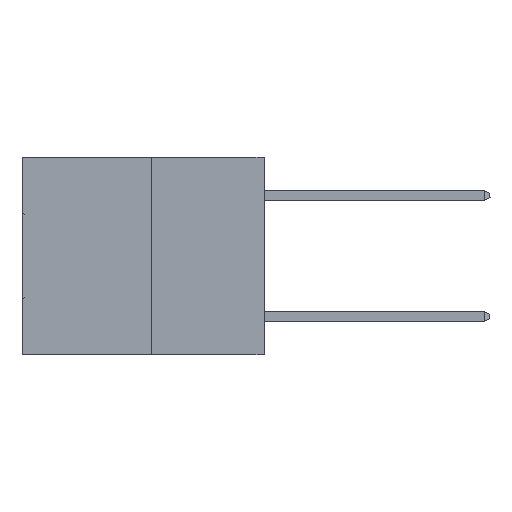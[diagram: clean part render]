
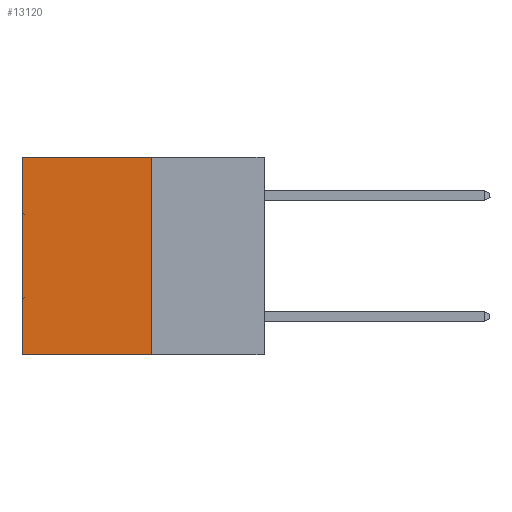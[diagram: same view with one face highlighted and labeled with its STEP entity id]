
A CAD part, left-side view. The second image highlights one B-rep face of the part: STEP entity #13120.
In plain terms, the highlighted planar face has unit normal (-1, 0, 0).
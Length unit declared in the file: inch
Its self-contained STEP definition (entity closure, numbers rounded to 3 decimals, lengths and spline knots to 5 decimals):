
#228 = CARTESIAN_POINT ( 'NONE',  ( 0.3165, 0.28, -0.49 ) ) ;
#1295 = FACE_OUTER_BOUND ( 'NONE', #20181, .T. ) ;
#1435 = VECTOR ( 'NONE', #20917, 39.37008 ) ;
#1850 = LINE ( 'NONE', #34299, #25041 ) ;
#3273 = VERTEX_POINT ( 'NONE', #21828 ) ;
#4884 = VERTEX_POINT ( 'NONE', #9350 ) ;
#6890 = LINE ( 'NONE', #12494, #13400 ) ;
#7121 = EDGE_CURVE ( 'NONE', #3273, #4884, #6890, .T. ) ;
#8091 = VECTOR ( 'NONE', #23873, 39.37008 ) ;
#8576 = VERTEX_POINT ( 'NONE', #11749 ) ;
#9350 = CARTESIAN_POINT ( 'NONE',  ( 0.3165, 0.6, -0.49 ) ) ;
#9595 = DIRECTION ( 'NONE',  ( 1., 0., 0. ) ) ;
#9751 = LINE ( 'NONE', #228, #1435 ) ;
#10992 = CARTESIAN_POINT ( 'NONE',  ( 0.3165, 0.28, -0.49 ) ) ;
#11749 = CARTESIAN_POINT ( 'NONE',  ( 0.3165, 0.28, 0. ) ) ;
#12494 = CARTESIAN_POINT ( 'NONE',  ( 0.3165, 0.6, -0.49 ) ) ;
#13120 = ADVANCED_FACE ( 'NONE', ( #1295 ), #26601, .F. ) ;
#13400 = VECTOR ( 'NONE', #15300, 39.37008 ) ;
#15300 = DIRECTION ( 'NONE',  ( 0., 0., -1. ) ) ;
#15886 = VERTEX_POINT ( 'NONE', #10992 ) ;
#16183 = EDGE_CURVE ( 'NONE', #15886, #4884, #9751, .T. ) ;
#17461 = DIRECTION ( 'NONE',  ( 0., 1., 0. ) ) ;
#18152 = DIRECTION ( 'NONE',  ( 0., 0., -1. ) ) ;
#20181 = EDGE_LOOP ( 'NONE', ( #36300, #35293, #36265, #30958 ) ) ;
#20768 = CARTESIAN_POINT ( 'NONE',  ( 0.3165, 0.28, -0.49 ) ) ;
#20917 = DIRECTION ( 'NONE',  ( 0., 1., 0. ) ) ;
#21828 = CARTESIAN_POINT ( 'NONE',  ( 0.3165, 0.6, 0. ) ) ;
#23873 = DIRECTION ( 'NONE',  ( 0., 0., -1. ) ) ;
#25041 = VECTOR ( 'NONE', #17461, 39.37008 ) ;
#25177 = LINE ( 'NONE', #32786, #8091 ) ;
#26601 = PLANE ( 'NONE',  #35656 ) ;
#30194 = EDGE_CURVE ( 'NONE', #8576, #15886, #25177, .T. ) ;
#30958 = ORIENTED_EDGE ( 'NONE', *, *, #32693, .T. ) ;
#32693 = EDGE_CURVE ( 'NONE', #8576, #3273, #1850, .T. ) ;
#32786 = CARTESIAN_POINT ( 'NONE',  ( 0.3165, 0.28, -0.49 ) ) ;
#34299 = CARTESIAN_POINT ( 'NONE',  ( 0.3165, 0.28, 0. ) ) ;
#35293 = ORIENTED_EDGE ( 'NONE', *, *, #16183, .F. ) ;
#35656 = AXIS2_PLACEMENT_3D ( 'NONE', #20768, #9595, #18152 ) ;
#36265 = ORIENTED_EDGE ( 'NONE', *, *, #30194, .F. ) ;
#36300 = ORIENTED_EDGE ( 'NONE', *, *, #7121, .T. ) ;
